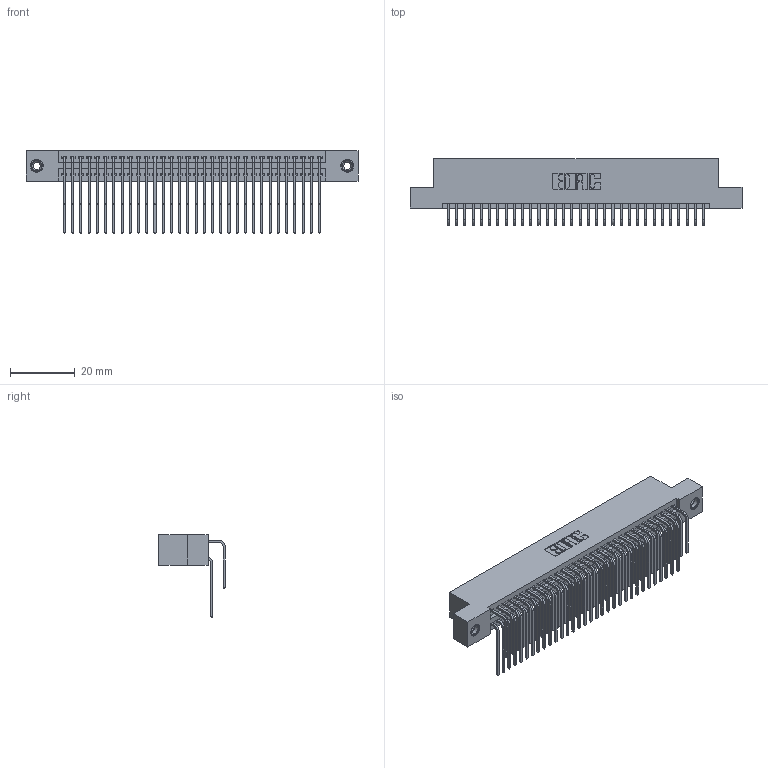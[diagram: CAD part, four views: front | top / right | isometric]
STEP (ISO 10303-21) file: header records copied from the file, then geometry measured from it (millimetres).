
FILE_DESCRIPTION (( 'STEP AP203' ), '1' );
FILE_NAME ('395-064-559-208.STEP', '2018-11-24T19:32:03', ( '' ), ( '' ), 'SwSTEP 2.0', 'SolidWorks 2016', '' );
FILE_SCHEMA (( 'CONFIG_CONTROL_DESIGN' ));
Length unit declared in the file: inch
Products named in the file (5): 345 Part_Flush Mounting Lugs - 0.156 Dia-TI; 345-292-001_558 559 Tail - 1; 345-250-001_345-250-003-102; 395-064-559-208; 345-292-001_559 Tail - 2
Assembly tree (67 placements, depth 2):
  395-064-559-208
    345 Part_Flush Mounting Lugs - 0.156 Dia-TI
    345-292-001_558 559 Tail - 1  x32
    345-292-001_559 Tail - 2  x32
    345-250-001_345-250-003-102  x2
Bounding box: 102.49 x 20.56 x 25.53 mm (x, y, z)
Volume: 10225.7 mm3; surface area: 16671.2 mm2
Topology: 67 solids, 67 shells, 3514 faces, 10397 edges, 6838 vertices
Faces by surface type: plane 2352, cylinder 1146, cone 12, torus 4
Entity records: 29292 total; most frequent: CARTESIAN_POINT 4946, ORIENTED_EDGE 4822, DIRECTION 4373, EDGE_CURVE 2411, LINE 2091, VECTOR 2091, VERTEX_POINT 1600, AXIS2_PLACEMENT_3D 1141
